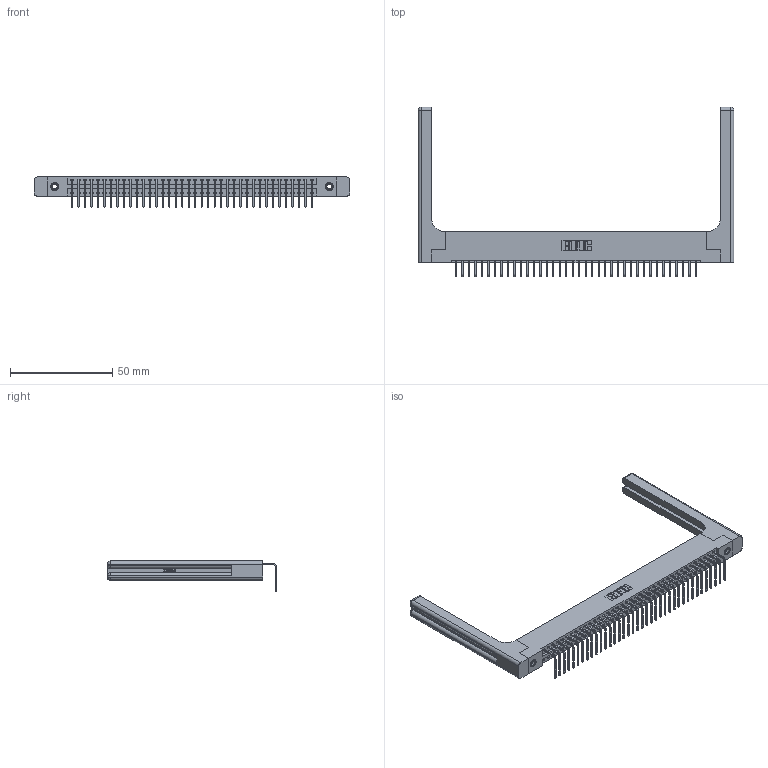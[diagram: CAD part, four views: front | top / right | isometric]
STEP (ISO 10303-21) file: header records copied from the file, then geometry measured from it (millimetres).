
FILE_DESCRIPTION (( 'STEP AP203' ), '1' );
FILE_NAME ('346-038-558-158.STEP', '2022-05-07T05:40:13', ( '' ), ( '' ), 'SwSTEP 2.0', 'SolidWorks 2020', '' );
FILE_SCHEMA (( 'CONFIG_CONTROL_DESIGN' ));
Length unit declared in the file: inch
Products named in the file (5): 346 Part_Flush Mounting Lugs - 0.156 Dia-TH; 346-220-058_345-220-058; 346-038-558-158; 345-250-001_345-250-001-102; 345-292-001_558 Tail - 2
Assembly tree (43 placements, depth 2):
  346-038-558-158
    346 Part_Flush Mounting Lugs - 0.156 Dia-TH
    345-292-001_558 Tail - 2  x38
    345-250-001_345-250-001-102  x2
    346-220-058_345-220-058  x2
Bounding box: 154.71 x 83.12 x 14.73 mm (x, y, z)
Volume: 22408.6 mm3; surface area: 24524.9 mm2
Topology: 43 solids, 43 shells, 2672 faces, 7947 edges, 5226 vertices
Faces by surface type: plane 1834, cylinder 778, bspline 36, cone 12, sphere 8, torus 4
Entity records: 29804 total; most frequent: CARTESIAN_POINT 6093, ORIENTED_EDGE 4860, DIRECTION 4310, EDGE_CURVE 2430, VECTOR 2054, LINE 2054, VERTEX_POINT 1610, AXIS2_PLACEMENT_3D 1128
